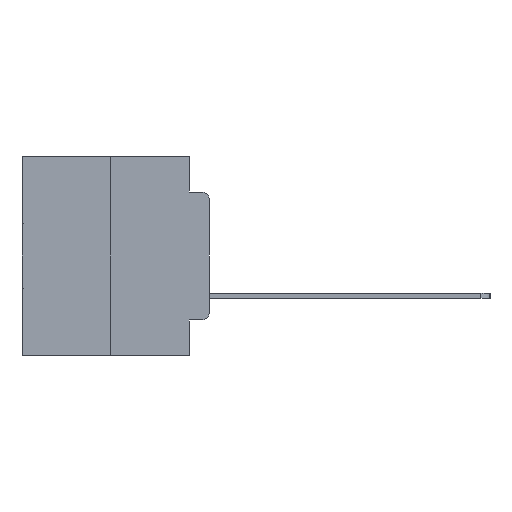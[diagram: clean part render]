
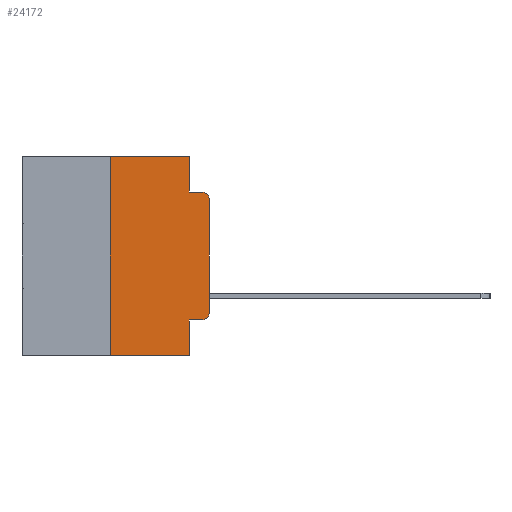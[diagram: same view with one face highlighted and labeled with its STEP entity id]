
A CAD part, left-side view. The second image highlights one B-rep face of the part: STEP entity #24172.
In plain terms, the highlighted planar face has unit normal (-1, 0, 0).
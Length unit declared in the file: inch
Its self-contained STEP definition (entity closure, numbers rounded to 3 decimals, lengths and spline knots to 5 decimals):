
#281 = ORIENTED_EDGE ( 'NONE', *, *, #13452, .F. ) ;
#429 = VECTOR ( 'NONE', #12679, 39.37008 ) ;
#833 = DIRECTION ( 'NONE',  ( 1., 0., 0. ) ) ;
#926 = CARTESIAN_POINT ( 'NONE',  ( 0., 0.25, 0. ) ) ;
#1031 = CARTESIAN_POINT ( 'NONE',  ( 0., 0.051, -0.5 ) ) ;
#1301 = CARTESIAN_POINT ( 'NONE',  ( 0., 0.473, -0.5 ) ) ;
#1694 = ORIENTED_EDGE ( 'NONE', *, *, #8032, .F. ) ;
#1718 = ORIENTED_EDGE ( 'NONE', *, *, #3213, .F. ) ;
#1952 = DIRECTION ( 'NONE',  ( 0., 0., 1. ) ) ;
#2348 = VERTEX_POINT ( 'NONE', #21810 ) ;
#2890 = DIRECTION ( 'NONE',  ( -1., 0., 0. ) ) ;
#3143 = CARTESIAN_POINT ( 'NONE',  ( 0., 0.02, -0.4115 ) ) ;
#3213 = EDGE_CURVE ( 'NONE', #11081, #2348, #24165, .T. ) ;
#3355 = EDGE_LOOP ( 'NONE', ( #18559, #7643, #281, #1718, #1694, #23869, #9835, #12530, #4711, #19546 ) ) ;
#3805 = DIRECTION ( 'NONE',  ( 0., 0., -1. ) ) ;
#3929 = VERTEX_POINT ( 'NONE', #21801 ) ;
#4250 = CARTESIAN_POINT ( 'NONE',  ( 0., 0.051, -0.0885 ) ) ;
#4711 = ORIENTED_EDGE ( 'NONE', *, *, #13501, .T. ) ;
#4764 = EDGE_CURVE ( 'NONE', #21461, #20966, #8917, .T. ) ;
#4786 = VERTEX_POINT ( 'NONE', #5663 ) ;
#4853 = EDGE_CURVE ( 'NONE', #21461, #24192, #16981, .T. ) ;
#4991 = VECTOR ( 'NONE', #26751, 39.37008 ) ;
#5663 = CARTESIAN_POINT ( 'NONE',  ( 0., 0., -0.1085 ) ) ;
#7314 = VECTOR ( 'NONE', #26308, 39.37008 ) ;
#7643 = ORIENTED_EDGE ( 'NONE', *, *, #18394, .T. ) ;
#8032 = EDGE_CURVE ( 'NONE', #20966, #11081, #26769, .T. ) ;
#8414 = AXIS2_PLACEMENT_3D ( 'NONE', #15963, #2890, #18141 ) ;
#8495 = DIRECTION ( 'NONE',  ( -1., 0., 0. ) ) ;
#8896 = CARTESIAN_POINT ( 'NONE',  ( 0., 0.051, -0.4115 ) ) ;
#8917 = LINE ( 'NONE', #926, #13920 ) ;
#9835 = ORIENTED_EDGE ( 'NONE', *, *, #4853, .T. ) ;
#10041 = LINE ( 'NONE', #25016, #13393 ) ;
#10973 = CARTESIAN_POINT ( 'NONE',  ( 0., 0.051, 0. ) ) ;
#11081 = VERTEX_POINT ( 'NONE', #10973 ) ;
#11240 = VECTOR ( 'NONE', #20608, 39.37008 ) ;
#11951 = AXIS2_PLACEMENT_3D ( 'NONE', #22529, #833, #24559 ) ;
#12530 = ORIENTED_EDGE ( 'NONE', *, *, #14937, .F. ) ;
#12679 = DIRECTION ( 'NONE',  ( 0., 0., 1. ) ) ;
#12802 = VECTOR ( 'NONE', #21583, 39.37008 ) ;
#13242 = CIRCLE ( 'NONE', #18328, 0.02 ) ;
#13393 = VECTOR ( 'NONE', #3805, 39.37008 ) ;
#13452 = EDGE_CURVE ( 'NONE', #2348, #14119, #25222, .T. ) ;
#13501 = EDGE_CURVE ( 'NONE', #22497, #26550, #19173, .T. ) ;
#13920 = VECTOR ( 'NONE', #1952, 39.37008 ) ;
#14119 = VERTEX_POINT ( 'NONE', #22503 ) ;
#14937 = EDGE_CURVE ( 'NONE', #22497, #24192, #10041, .T. ) ;
#14978 = EDGE_CURVE ( 'NONE', #3929, #4786, #17228, .T. ) ;
#15303 = CIRCLE ( 'NONE', #8414, 0.02 ) ;
#15963 = CARTESIAN_POINT ( 'NONE',  ( 0., 0.02, -0.1085 ) ) ;
#16043 = CARTESIAN_POINT ( 'NONE',  ( 0., 0.25, -0.5 ) ) ;
#16981 = LINE ( 'NONE', #1301, #11240 ) ;
#17228 = LINE ( 'NONE', #27217, #429 ) ;
#17256 = DIRECTION ( 'NONE',  ( 0., -1., 0. ) ) ;
#18141 = DIRECTION ( 'NONE',  ( 0., 0., -1. ) ) ;
#18328 = AXIS2_PLACEMENT_3D ( 'NONE', #21198, #8495, #23298 ) ;
#18394 = EDGE_CURVE ( 'NONE', #4786, #14119, #15303, .T. ) ;
#18559 = ORIENTED_EDGE ( 'NONE', *, *, #14978, .T. ) ;
#18567 = CARTESIAN_POINT ( 'NONE',  ( 0., 0.051, -0.4115 ) ) ;
#19173 = LINE ( 'NONE', #8896, #12802 ) ;
#19310 = EDGE_CURVE ( 'NONE', #26550, #3929, #13242, .T. ) ;
#19546 = ORIENTED_EDGE ( 'NONE', *, *, #19310, .T. ) ;
#20432 = PLANE ( 'NONE',  #11951 ) ;
#20608 = DIRECTION ( 'NONE',  ( 0., -1., 0. ) ) ;
#20966 = VERTEX_POINT ( 'NONE', #25017 ) ;
#21198 = CARTESIAN_POINT ( 'NONE',  ( 0., 0.02, -0.3915 ) ) ;
#21461 = VERTEX_POINT ( 'NONE', #16043 ) ;
#21583 = DIRECTION ( 'NONE',  ( 0., -1., 0. ) ) ;
#21801 = CARTESIAN_POINT ( 'NONE',  ( 0., 0., -0.3915 ) ) ;
#21810 = CARTESIAN_POINT ( 'NONE',  ( 0., 0.051, -0.0885 ) ) ;
#22497 = VERTEX_POINT ( 'NONE', #18567 ) ;
#22503 = CARTESIAN_POINT ( 'NONE',  ( 0., 0.02, -0.0885 ) ) ;
#22529 = CARTESIAN_POINT ( 'NONE',  ( 0., 0.473, 0. ) ) ;
#22713 = CARTESIAN_POINT ( 'NONE',  ( 0., 0.473, 0. ) ) ;
#23105 = FACE_OUTER_BOUND ( 'NONE', #3355, .T. ) ;
#23298 = DIRECTION ( 'NONE',  ( 0., 0., -1. ) ) ;
#23601 = CARTESIAN_POINT ( 'NONE',  ( 0., 0.051, 0. ) ) ;
#23869 = ORIENTED_EDGE ( 'NONE', *, *, #4764, .F. ) ;
#24165 = LINE ( 'NONE', #23601, #7314 ) ;
#24172 = ADVANCED_FACE ( 'NONE', ( #23105 ), #20432, .F. ) ;
#24192 = VERTEX_POINT ( 'NONE', #1031 ) ;
#24559 = DIRECTION ( 'NONE',  ( 0., 0., -1. ) ) ;
#24588 = VECTOR ( 'NONE', #17256, 39.37008 ) ;
#25016 = CARTESIAN_POINT ( 'NONE',  ( 0., 0.051, 0. ) ) ;
#25017 = CARTESIAN_POINT ( 'NONE',  ( 0., 0.25, 0. ) ) ;
#25222 = LINE ( 'NONE', #4250, #24588 ) ;
#26308 = DIRECTION ( 'NONE',  ( 0., 0., -1. ) ) ;
#26550 = VERTEX_POINT ( 'NONE', #3143 ) ;
#26751 = DIRECTION ( 'NONE',  ( 0., -1., 0. ) ) ;
#26769 = LINE ( 'NONE', #22713, #4991 ) ;
#27217 = CARTESIAN_POINT ( 'NONE',  ( 0., 0., 0. ) ) ;
